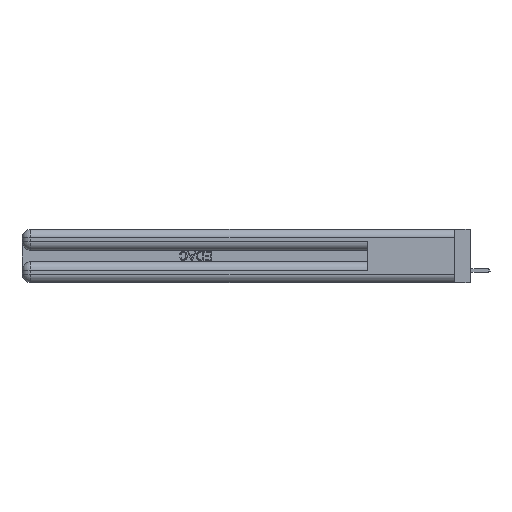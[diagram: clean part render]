
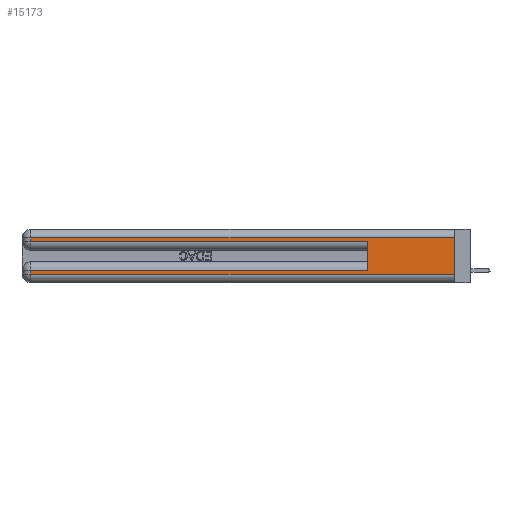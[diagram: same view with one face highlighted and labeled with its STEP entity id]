
A CAD part, left-side view. The second image highlights one B-rep face of the part: STEP entity #15173.
In plain terms, the highlighted planar face has unit normal (-1, 0, 0).
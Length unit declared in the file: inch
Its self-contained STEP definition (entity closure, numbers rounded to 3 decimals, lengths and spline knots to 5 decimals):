
#741 = VECTOR ( 'NONE', #41506, 39.37008 ) ;
#1110 = PLANE ( 'NONE',  #22671 ) ;
#1379 = CARTESIAN_POINT ( 'NONE',  ( 0., 0.6, 0.085 ) ) ;
#1415 = VERTEX_POINT ( 'NONE', #8219 ) ;
#2102 = DIRECTION ( 'NONE',  ( 0., 0., -1. ) ) ;
#2162 = LINE ( 'NONE', #8419, #19780 ) ;
#2666 = EDGE_CURVE ( 'NONE', #11625, #29699, #40339, .T. ) ;
#4129 = ORIENTED_EDGE ( 'NONE', *, *, #17939, .F. ) ;
#4240 = CARTESIAN_POINT ( 'NONE',  ( 0., 0., 0.37 ) ) ;
#5718 = DIRECTION ( 'NONE',  ( 0., -1., 0. ) ) ;
#6155 = CARTESIAN_POINT ( 'NONE',  ( 0., 0., 0.06 ) ) ;
#6575 = VERTEX_POINT ( 'NONE', #26087 ) ;
#6834 = LINE ( 'NONE', #6155, #741 ) ;
#7591 = EDGE_CURVE ( 'NONE', #23103, #1415, #6834, .T. ) ;
#8219 = CARTESIAN_POINT ( 'NONE',  ( 0., 0., 0.06 ) ) ;
#8419 = CARTESIAN_POINT ( 'NONE',  ( 0., 2.94, 0.37 ) ) ;
#9283 = CARTESIAN_POINT ( 'NONE',  ( 0., 0., 0.31 ) ) ;
#10585 = DIRECTION ( 'NONE',  ( 1., 0., 0. ) ) ;
#11588 = EDGE_LOOP ( 'NONE', ( #4129, #23066, #28547, #12771, #29426, #36960, #15072, #41620 ) ) ;
#11625 = VERTEX_POINT ( 'NONE', #1379 ) ;
#11894 = DIRECTION ( 'NONE',  ( 0., 0., -1. ) ) ;
#12771 = ORIENTED_EDGE ( 'NONE', *, *, #38183, .T. ) ;
#13486 = EDGE_CURVE ( 'NONE', #11625, #16534, #36302, .T. ) ;
#14634 = DIRECTION ( 'NONE',  ( 0., 1., 0. ) ) ;
#15072 = ORIENTED_EDGE ( 'NONE', *, *, #19202, .T. ) ;
#15173 = ADVANCED_FACE ( 'NONE', ( #35188 ), #1110, .F. ) ;
#16534 = VERTEX_POINT ( 'NONE', #20840 ) ;
#16871 = LINE ( 'NONE', #30513, #30532 ) ;
#17750 = VERTEX_POINT ( 'NONE', #23172 ) ;
#17939 = EDGE_CURVE ( 'NONE', #17750, #1415, #29557, .T. ) ;
#18692 = CARTESIAN_POINT ( 'NONE',  ( 0., 0., 0.285 ) ) ;
#18963 = EDGE_CURVE ( 'NONE', #17750, #6575, #28089, .T. ) ;
#19109 = LINE ( 'NONE', #18692, #21103 ) ;
#19202 = EDGE_CURVE ( 'NONE', #29699, #23103, #16871, .T. ) ;
#19780 = VECTOR ( 'NONE', #2102, 39.37008 ) ;
#20133 = VERTEX_POINT ( 'NONE', #37465 ) ;
#20840 = CARTESIAN_POINT ( 'NONE',  ( 0., 0.6, 0.285 ) ) ;
#21103 = VECTOR ( 'NONE', #5718, 39.37008 ) ;
#21106 = CARTESIAN_POINT ( 'NONE',  ( 0., 2.94, 0.06 ) ) ;
#22643 = VECTOR ( 'NONE', #37472, 39.37008 ) ;
#22671 = AXIS2_PLACEMENT_3D ( 'NONE', #4240, #10585, #33170 ) ;
#23066 = ORIENTED_EDGE ( 'NONE', *, *, #18963, .T. ) ;
#23103 = VERTEX_POINT ( 'NONE', #21106 ) ;
#23172 = CARTESIAN_POINT ( 'NONE',  ( 0., 0., 0.31 ) ) ;
#24268 = CARTESIAN_POINT ( 'NONE',  ( 0., 0.6, 0.145 ) ) ;
#24436 = CARTESIAN_POINT ( 'NONE',  ( 0., 0., 0.37 ) ) ;
#25305 = EDGE_CURVE ( 'NONE', #6575, #20133, #2162, .T. ) ;
#25964 = DIRECTION ( 'NONE',  ( 0., 0., -1. ) ) ;
#26048 = VECTOR ( 'NONE', #25964, 39.37008 ) ;
#26087 = CARTESIAN_POINT ( 'NONE',  ( 0., 2.94, 0.31 ) ) ;
#28089 = LINE ( 'NONE', #9283, #38226 ) ;
#28547 = ORIENTED_EDGE ( 'NONE', *, *, #25305, .T. ) ;
#29426 = ORIENTED_EDGE ( 'NONE', *, *, #13486, .F. ) ;
#29557 = LINE ( 'NONE', #24436, #26048 ) ;
#29699 = VERTEX_POINT ( 'NONE', #38483 ) ;
#30513 = CARTESIAN_POINT ( 'NONE',  ( 0., 2.94, 0.37 ) ) ;
#30532 = VECTOR ( 'NONE', #11894, 39.37008 ) ;
#32241 = VECTOR ( 'NONE', #14634, 39.37008 ) ;
#33170 = DIRECTION ( 'NONE',  ( 0., 0., -1. ) ) ;
#35188 = FACE_OUTER_BOUND ( 'NONE', #11588, .T. ) ;
#36302 = LINE ( 'NONE', #24268, #22643 ) ;
#36337 = DIRECTION ( 'NONE',  ( 0., 1., 0. ) ) ;
#36960 = ORIENTED_EDGE ( 'NONE', *, *, #2666, .T. ) ;
#37107 = CARTESIAN_POINT ( 'NONE',  ( 0., 0., 0.085 ) ) ;
#37465 = CARTESIAN_POINT ( 'NONE',  ( 0., 2.94, 0.285 ) ) ;
#37472 = DIRECTION ( 'NONE',  ( 0., 0., 1. ) ) ;
#38183 = EDGE_CURVE ( 'NONE', #20133, #16534, #19109, .T. ) ;
#38226 = VECTOR ( 'NONE', #36337, 39.37008 ) ;
#38483 = CARTESIAN_POINT ( 'NONE',  ( 0., 2.94, 0.085 ) ) ;
#40339 = LINE ( 'NONE', #37107, #32241 ) ;
#41506 = DIRECTION ( 'NONE',  ( 0., -1., 0. ) ) ;
#41620 = ORIENTED_EDGE ( 'NONE', *, *, #7591, .T. ) ;
